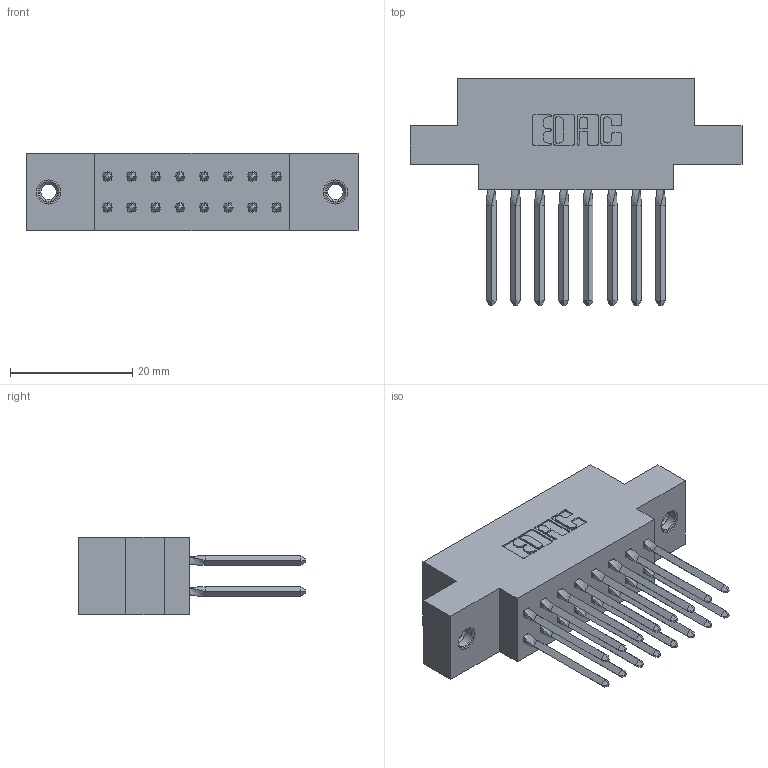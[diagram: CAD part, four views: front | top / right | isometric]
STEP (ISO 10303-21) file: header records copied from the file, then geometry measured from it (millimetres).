
FILE_DESCRIPTION (( 'STEP AP203' ), '1' );
FILE_NAME ('317-016-542-807.STEP', '2020-02-27T15:27:39', ( '' ), ( '' ), 'SwSTEP 2.0', 'SolidWorks 2016', '' );
FILE_SCHEMA (( 'CONFIG_CONTROL_DESIGN' ));
Length unit declared in the file: inch
Products named in the file (4): 317-016-542-807; 345-250-001_345-250-005-103; 317-290-003_542; 317 Part_.156 Dia - TI
Assembly tree (19 placements, depth 2):
  317-016-542-807
    317 Part_.156 Dia - TI
    317-290-003_542  x16
    345-250-001_345-250-005-103  x2
Bounding box: 54.41 x 37.34 x 12.7 mm (x, y, z)
Volume: 7820.9 mm3; surface area: 9821.1 mm2
Topology: 19 solids, 19 shells, 1074 faces, 2971 edges, 1898 vertices
Faces by surface type: plane 826, cylinder 168, bspline 64, cone 12, torus 4
Entity records: 16510 total; most frequent: CARTESIAN_POINT 3096, ORIENTED_EDGE 2752, DIRECTION 2414, EDGE_CURVE 1376, VECTOR 1186, LINE 1186, VERTEX_POINT 908, AXIS2_PLACEMENT_3D 614
